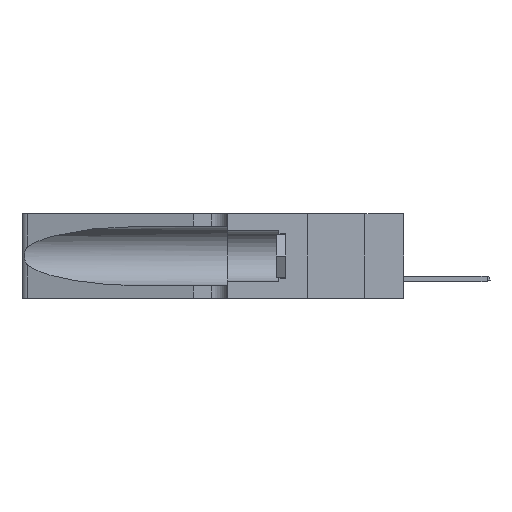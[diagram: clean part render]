
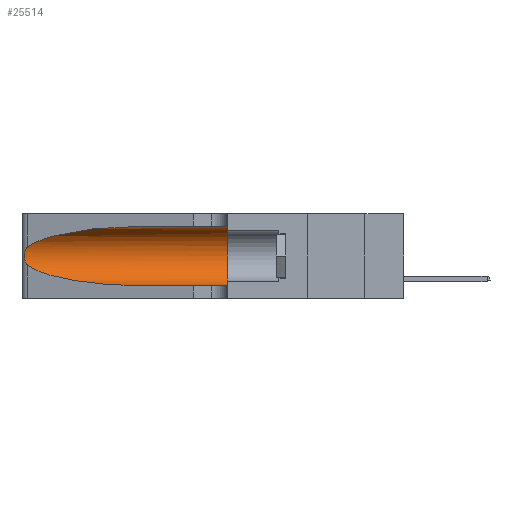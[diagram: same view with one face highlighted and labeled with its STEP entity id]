
A CAD part, left-side view. The second image highlights one B-rep face of the part: STEP entity #25514.
In plain terms, the highlighted cylindrical face has radius 3.308 mm (diameter 6.617 mm), a partial arc.
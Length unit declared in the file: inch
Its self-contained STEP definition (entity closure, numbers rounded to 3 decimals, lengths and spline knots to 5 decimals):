
#7 = DIRECTION ( 'NONE',  ( 0., 0., -1. ) ) ;
#46 = ORIENTED_EDGE ( 'NONE', *, *, #786, .T. ) ;
#574 = CARTESIAN_POINT ( 'NONE',  ( 0.25856, 1.23593, 0.16098 ) ) ;
#662 = VECTOR ( 'NONE', #5066, 39.37008 ) ;
#761 = ORIENTED_EDGE ( 'NONE', *, *, #24230, .F. ) ;
#786 = EDGE_CURVE ( 'NONE', #7468, #17803, #10319, .T. ) ;
#884 = ORIENTED_EDGE ( 'NONE', *, *, #7161, .T. ) ;
#1132 = CARTESIAN_POINT ( 'NONE',  ( 0.1305, 0.35, 0.05475 ) ) ;
#1844 = CARTESIAN_POINT ( 'NONE',  ( 0.1305, 0.35, 0.185 ) ) ;
#2525 = FACE_OUTER_BOUND ( 'NONE', #15453, .T. ) ;
#2770 = CARTESIAN_POINT ( 'NONE',  ( 0.1305, 0.72297, 0.31525 ) ) ;
#2905 = B_SPLINE_CURVE_WITH_KNOTS ( 'NONE', 3,
 ( #7395, #8129, #12892, #17275, #22284, #7891, #15424, #17911, #27687, #574, #10619, #20275, #5553, #5665 ),
 .UNSPECIFIED., .F., .F.,
 ( 4, 2, 2, 2, 2, 2, 4 ),
 ( 0., 0.00027, 0.00053, 0.00107, 0.0016, 0.00187, 0.00214 ),
 .UNSPECIFIED. ) ;
#2963 = VERTEX_POINT ( 'NONE', #30188 ) ;
#2993 = VERTEX_POINT ( 'NONE', #10801 ) ;
#3419 = VERTEX_POINT ( 'NONE', #25228 ) ;
#3836 = CARTESIAN_POINT ( 'NONE',  ( 0.1305, 1.61858, 0.31525 ) ) ;
#5066 = DIRECTION ( 'NONE',  ( 0., -1., 0. ) ) ;
#5429 = CARTESIAN_POINT ( 'NONE',  ( 0.1305, 1.61858, 0.05475 ) ) ;
#5553 = CARTESIAN_POINT ( 'NONE',  ( 0.25555, 1.22993, 0.14849 ) ) ;
#5665 = CARTESIAN_POINT ( 'NONE',  ( 0.25487, 1.22718, 0.14631 ) ) ;
#6012 = ORIENTED_EDGE ( 'NONE', *, *, #20395, .F. ) ;
#6146 = VERTEX_POINT ( 'NONE', #8721 ) ;
#7161 = EDGE_CURVE ( 'NONE', #2993, #2963, #2905, .T. ) ;
#7395 = CARTESIAN_POINT ( 'NONE',  ( 0.25487, 1.22718, 0.22369 ) ) ;
#7468 = VERTEX_POINT ( 'NONE', #27671 ) ;
#7891 = CARTESIAN_POINT ( 'NONE',  ( 0.26018, 1.23835, 0.19895 ) ) ;
#8129 = CARTESIAN_POINT ( 'NONE',  ( 0.25555, 1.22994, 0.2215 ) ) ;
#8476 = CARTESIAN_POINT ( 'NONE',  ( 0.18966, 0.96281, 0.05475 ) ) ;
#8721 = CARTESIAN_POINT ( 'NONE',  ( 0.1305, 0.35, 0.31525 ) ) ;
#9694 =( BOUNDED_CURVE ( )  B_SPLINE_CURVE ( 3, ( #28399, #20989, #8476, #25761 ),
 .UNSPECIFIED., .F., .F. ) 
 B_SPLINE_CURVE_WITH_KNOTS ( ( 4, 4 ),
 ( 3.44316, 4.71239 ),
 .UNSPECIFIED. ) 
 CURVE ( )  GEOMETRIC_REPRESENTATION_ITEM ( )  RATIONAL_B_SPLINE_CURVE ( ( 1., 0.87, 0.87, 1. ) ) 
 REPRESENTATION_ITEM ( '' )  );
#10319 = LINE ( 'NONE', #5429, #662 ) ;
#10619 = CARTESIAN_POINT ( 'NONE',  ( 0.25789, 1.23486, 0.15765 ) ) ;
#10801 = CARTESIAN_POINT ( 'NONE',  ( 0.25487, 1.22718, 0.22369 ) ) ;
#11251 = AXIS2_PLACEMENT_3D ( 'NONE', #14731, #27377, #7 ) ;
#12372 = ORIENTED_EDGE ( 'NONE', *, *, #28117, .T. ) ;
#12892 = CARTESIAN_POINT ( 'NONE',  ( 0.25639, 1.23184, 0.21858 ) ) ;
#13047 =( BOUNDED_CURVE ( )  B_SPLINE_CURVE ( 3, ( #2770, #19808, #29961, #25001 ),
 .UNSPECIFIED., .F., .T. ) 
 B_SPLINE_CURVE_WITH_KNOTS ( ( 4, 4 ),
 ( 1.5708, 2.84003 ),
 .UNSPECIFIED. ) 
 CURVE ( )  GEOMETRIC_REPRESENTATION_ITEM ( )  RATIONAL_B_SPLINE_CURVE ( ( 1., 0.87, 0.87, 1. ) ) 
 REPRESENTATION_ITEM ( '' )  );
#14494 = CYLINDRICAL_SURFACE ( 'NONE', #11251, 0.13025 ) ;
#14731 = CARTESIAN_POINT ( 'NONE',  ( 0.1305, 1.61858, 0.185 ) ) ;
#15424 = CARTESIAN_POINT ( 'NONE',  ( 0.26075, 1.23896, 0.19203 ) ) ;
#15453 = EDGE_LOOP ( 'NONE', ( #12372, #884, #16604, #46, #6012, #761 ) ) ;
#16604 = ORIENTED_EDGE ( 'NONE', *, *, #17843, .T. ) ;
#17275 = CARTESIAN_POINT ( 'NONE',  ( 0.25787, 1.23484, 0.2124 ) ) ;
#17424 = CIRCLE ( 'NONE', #21487, 0.13025 ) ;
#17568 = VECTOR ( 'NONE', #18452, 39.37008 ) ;
#17803 = VERTEX_POINT ( 'NONE', #1132 ) ;
#17843 = EDGE_CURVE ( 'NONE', #2963, #7468, #9694, .T. ) ;
#17911 = CARTESIAN_POINT ( 'NONE',  ( 0.26075, 1.23896, 0.178 ) ) ;
#18452 = DIRECTION ( 'NONE',  ( 0., -1., 0. ) ) ;
#18751 = DIRECTION ( 'NONE',  ( 0., 0., 1. ) ) ;
#19808 = CARTESIAN_POINT ( 'NONE',  ( 0.18966, 0.96281, 0.31525 ) ) ;
#20275 = CARTESIAN_POINT ( 'NONE',  ( 0.25639, 1.23186, 0.15144 ) ) ;
#20395 = EDGE_CURVE ( 'NONE', #6146, #17803, #17424, .T. ) ;
#20989 = CARTESIAN_POINT ( 'NONE',  ( 0.2373, 1.15595, 0.08982 ) ) ;
#21487 = AXIS2_PLACEMENT_3D ( 'NONE', #1844, #31199, #18751 ) ;
#22284 = CARTESIAN_POINT ( 'NONE',  ( 0.25854, 1.2359, 0.20912 ) ) ;
#22643 = LINE ( 'NONE', #3836, #17568 ) ;
#24230 = EDGE_CURVE ( 'NONE', #3419, #6146, #22643, .T. ) ;
#25001 = CARTESIAN_POINT ( 'NONE',  ( 0.25487, 1.22718, 0.22369 ) ) ;
#25228 = CARTESIAN_POINT ( 'NONE',  ( 0.1305, 0.72297, 0.31525 ) ) ;
#25514 = ADVANCED_FACE ( 'NONE', ( #2525 ), #14494, .F. ) ;
#25761 = CARTESIAN_POINT ( 'NONE',  ( 0.1305, 0.72297, 0.05475 ) ) ;
#27377 = DIRECTION ( 'NONE',  ( 0., -1., 0. ) ) ;
#27671 = CARTESIAN_POINT ( 'NONE',  ( 0.1305, 0.72297, 0.05475 ) ) ;
#27687 = CARTESIAN_POINT ( 'NONE',  ( 0.26017, 1.23833, 0.17102 ) ) ;
#28117 = EDGE_CURVE ( 'NONE', #3419, #2993, #13047, .T. ) ;
#28399 = CARTESIAN_POINT ( 'NONE',  ( 0.25487, 1.22718, 0.14631 ) ) ;
#29961 = CARTESIAN_POINT ( 'NONE',  ( 0.2373, 1.15595, 0.28018 ) ) ;
#30188 = CARTESIAN_POINT ( 'NONE',  ( 0.25487, 1.22718, 0.14631 ) ) ;
#31199 = DIRECTION ( 'NONE',  ( 0., 1., 0. ) ) ;
